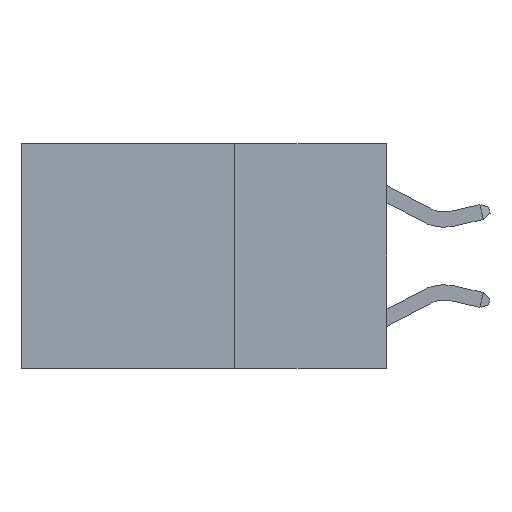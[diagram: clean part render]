
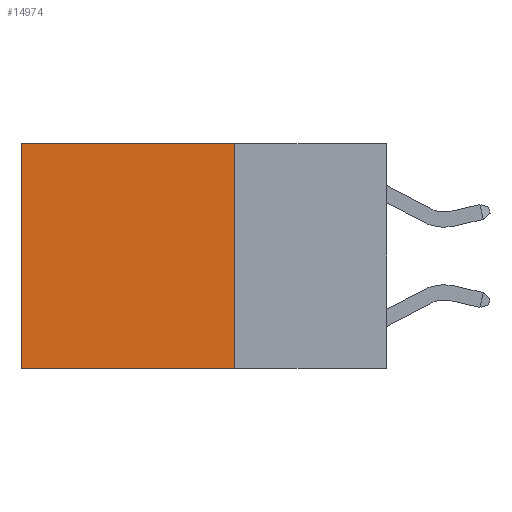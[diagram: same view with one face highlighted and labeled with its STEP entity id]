
A CAD part, left-side view. The second image highlights one B-rep face of the part: STEP entity #14974.
In plain terms, the highlighted planar face has unit normal (-1, 0, 0).
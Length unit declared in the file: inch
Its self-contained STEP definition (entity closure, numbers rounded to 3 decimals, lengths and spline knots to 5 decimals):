
#432 = ORIENTED_EDGE ( 'NONE', *, *, #8942, .T. ) ;
#2068 = CARTESIAN_POINT ( 'NONE',  ( 0.2625, 0.25, 0. ) ) ;
#2129 = PLANE ( 'NONE',  #18765 ) ;
#2575 = LINE ( 'NONE', #4963, #15508 ) ;
#3809 = LINE ( 'NONE', #2068, #16206 ) ;
#3868 = CARTESIAN_POINT ( 'NONE',  ( 0.2625, 0.25, 0. ) ) ;
#4370 = EDGE_CURVE ( 'NONE', #6494, #4504, #7655, .T. ) ;
#4480 = CARTESIAN_POINT ( 'NONE',  ( 0.2625, 0.25, -0.37 ) ) ;
#4504 = VERTEX_POINT ( 'NONE', #7449 ) ;
#4679 = CARTESIAN_POINT ( 'NONE',  ( 0.2625, 0.25, -0.37 ) ) ;
#4963 = CARTESIAN_POINT ( 'NONE',  ( 0.2625, 0.25, 0. ) ) ;
#5867 = VECTOR ( 'NONE', #8042, 39.37008 ) ;
#6494 = VERTEX_POINT ( 'NONE', #11430 ) ;
#6618 = DIRECTION ( 'NONE',  ( 0., 0., -1. ) ) ;
#7211 = FACE_OUTER_BOUND ( 'NONE', #7890, .T. ) ;
#7257 = DIRECTION ( 'NONE',  ( 0., 0., -1. ) ) ;
#7449 = CARTESIAN_POINT ( 'NONE',  ( 0.2625, 0.6, -0.37 ) ) ;
#7655 = LINE ( 'NONE', #12144, #16103 ) ;
#7890 = EDGE_LOOP ( 'NONE', ( #11087, #9972, #17240, #432 ) ) ;
#8042 = DIRECTION ( 'NONE',  ( 0., 1., 0. ) ) ;
#8710 = VERTEX_POINT ( 'NONE', #13243 ) ;
#8942 = EDGE_CURVE ( 'NONE', #8710, #6494, #3809, .T. ) ;
#9972 = ORIENTED_EDGE ( 'NONE', *, *, #15316, .F. ) ;
#11087 = ORIENTED_EDGE ( 'NONE', *, *, #4370, .T. ) ;
#11430 = CARTESIAN_POINT ( 'NONE',  ( 0.2625, 0.6, 0. ) ) ;
#12144 = CARTESIAN_POINT ( 'NONE',  ( 0.2625, 0.6, 0. ) ) ;
#13243 = CARTESIAN_POINT ( 'NONE',  ( 0.2625, 0.25, 0. ) ) ;
#14974 = ADVANCED_FACE ( 'NONE', ( #7211 ), #2129, .F. ) ;
#15316 = EDGE_CURVE ( 'NONE', #16638, #4504, #19568, .T. ) ;
#15508 = VECTOR ( 'NONE', #6618, 39.37008 ) ;
#15562 = DIRECTION ( 'NONE',  ( 0., 1., 0. ) ) ;
#15617 = DIRECTION ( 'NONE',  ( 0., 0., -1. ) ) ;
#16103 = VECTOR ( 'NONE', #15617, 39.37008 ) ;
#16206 = VECTOR ( 'NONE', #15562, 39.37008 ) ;
#16638 = VERTEX_POINT ( 'NONE', #4480 ) ;
#17240 = ORIENTED_EDGE ( 'NONE', *, *, #17285, .F. ) ;
#17285 = EDGE_CURVE ( 'NONE', #8710, #16638, #2575, .T. ) ;
#17441 = DIRECTION ( 'NONE',  ( 1., 0., 0. ) ) ;
#18765 = AXIS2_PLACEMENT_3D ( 'NONE', #3868, #17441, #7257 ) ;
#19568 = LINE ( 'NONE', #4679, #5867 ) ;
